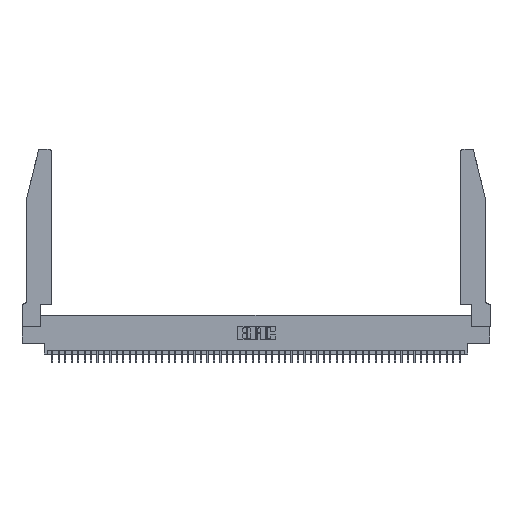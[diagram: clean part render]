
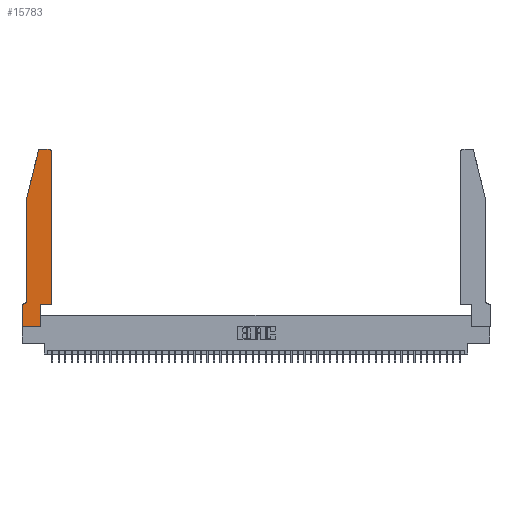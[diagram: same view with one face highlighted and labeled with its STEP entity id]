
A CAD part, top view. The second image highlights one B-rep face of the part: STEP entity #15783.
In plain terms, the highlighted planar face has unit normal (0, 0, 1).
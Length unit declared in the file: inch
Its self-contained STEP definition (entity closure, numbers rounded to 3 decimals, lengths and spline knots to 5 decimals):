
#323 = CARTESIAN_POINT ( 'NONE',  ( 0.284, 2.72, 0.37 ) ) ;
#986 = ORIENTED_EDGE ( 'NONE', *, *, #10492, .T. ) ;
#1044 = EDGE_CURVE ( 'NONE', #39456, #3815, #16891, .T. ) ;
#1156 = VERTEX_POINT ( 'NONE', #30139 ) ;
#1580 = CARTESIAN_POINT ( 'NONE',  ( 0.4505, 2.72, 0.37 ) ) ;
#1683 = CARTESIAN_POINT ( 'NONE',  ( 0.0755, 0.35, 0.37 ) ) ;
#2139 = AXIS2_PLACEMENT_3D ( 'NONE', #43723, #15956, #23377 ) ;
#3011 = PLANE ( 'NONE',  #17793 ) ;
#3158 = VERTEX_POINT ( 'NONE', #9696 ) ;
#3815 = VERTEX_POINT ( 'NONE', #37715 ) ;
#4300 = DIRECTION ( 'NONE',  ( 0., 0., 1. ) ) ;
#5509 = ORIENTED_EDGE ( 'NONE', *, *, #23324, .T. ) ;
#5514 = CIRCLE ( 'NONE', #7210, 0.03 ) ;
#6064 = EDGE_CURVE ( 'NONE', #20552, #37016, #24253, .T. ) ;
#7210 = AXIS2_PLACEMENT_3D ( 'NONE', #323, #4300, #49679 ) ;
#9147 = VERTEX_POINT ( 'NONE', #23112 ) ;
#9696 = CARTESIAN_POINT ( 'NONE',  ( 0.2865, 0.35, 0.37 ) ) ;
#9889 = ORIENTED_EDGE ( 'NONE', *, *, #6064, .T. ) ;
#10321 = VECTOR ( 'NONE', #38450, 39.37008 ) ;
#10492 = EDGE_CURVE ( 'NONE', #1156, #16856, #13989, .T. ) ;
#10498 = CARTESIAN_POINT ( 'NONE',  ( 0.4505, 0.35, 0.37 ) ) ;
#11010 = CARTESIAN_POINT ( 'NONE',  ( 0.2605, 2.75, 0.37 ) ) ;
#11026 = CARTESIAN_POINT ( 'NONE',  ( 0., 0., 0.37 ) ) ;
#11160 = ORIENTED_EDGE ( 'NONE', *, *, #1044, .T. ) ;
#12332 = ORIENTED_EDGE ( 'NONE', *, *, #48215, .T. ) ;
#13614 = VECTOR ( 'NONE', #44052, 39.37008 ) ;
#13898 = LINE ( 'NONE', #26039, #33734 ) ;
#13989 = CIRCLE ( 'NONE', #2139, 0.07 ) ;
#14153 = DIRECTION ( 'NONE',  ( -0.239, -0.971, 0. ) ) ;
#14894 = LINE ( 'NONE', #46168, #40842 ) ;
#15067 = ORIENTED_EDGE ( 'NONE', *, *, #27003, .T. ) ;
#15783 = ADVANCED_FACE ( 'NONE', ( #51404 ), #3011, .T. ) ;
#15956 = DIRECTION ( 'NONE',  ( 0., 0., -1. ) ) ;
#16856 = VERTEX_POINT ( 'NONE', #41423 ) ;
#16891 = CIRCLE ( 'NONE', #51468, 0.03 ) ;
#17680 = CARTESIAN_POINT ( 'NONE',  ( 0.2865, 0., 0.37 ) ) ;
#17793 = AXIS2_PLACEMENT_3D ( 'NONE', #30794, #35275, #31304 ) ;
#20552 = VERTEX_POINT ( 'NONE', #32306 ) ;
#21447 = VECTOR ( 'NONE', #27969, 39.37008 ) ;
#21716 = EDGE_CURVE ( 'NONE', #3158, #40963, #14894, .T. ) ;
#22412 = VERTEX_POINT ( 'NONE', #17680 ) ;
#22620 = VECTOR ( 'NONE', #14153, 39.37008 ) ;
#23112 = CARTESIAN_POINT ( 'NONE',  ( 0.0755, 2., 0.37 ) ) ;
#23324 = EDGE_CURVE ( 'NONE', #40963, #39456, #29226, .T. ) ;
#23377 = DIRECTION ( 'NONE',  ( -1., 0., 0. ) ) ;
#23760 = EDGE_CURVE ( 'NONE', #29981, #45880, #5514, .T. ) ;
#24253 = LINE ( 'NONE', #27253, #45060 ) ;
#24928 = VECTOR ( 'NONE', #45865, 39.37008 ) ;
#26039 = CARTESIAN_POINT ( 'NONE',  ( 0.0755, 2., 0.37 ) ) ;
#26827 = ORIENTED_EDGE ( 'NONE', *, *, #31838, .T. ) ;
#27003 = EDGE_CURVE ( 'NONE', #9147, #1156, #13898, .T. ) ;
#27135 = LINE ( 'NONE', #11010, #13614 ) ;
#27253 = CARTESIAN_POINT ( 'NONE',  ( 0., 0., 0.37 ) ) ;
#27969 = DIRECTION ( 'NONE',  ( 0., 1., 0. ) ) ;
#29226 = LINE ( 'NONE', #41891, #24928 ) ;
#29630 = DIRECTION ( 'NONE',  ( 0., 0., 1. ) ) ;
#29981 = VERTEX_POINT ( 'NONE', #41288 ) ;
#30015 = LINE ( 'NONE', #42165, #22620 ) ;
#30139 = CARTESIAN_POINT ( 'NONE',  ( 0.0755, 0.42, 0.37 ) ) ;
#30794 = CARTESIAN_POINT ( 'NONE',  ( 0., 0.35, 0.37 ) ) ;
#31000 = DIRECTION ( 'NONE',  ( 1., 0., 0. ) ) ;
#31304 = DIRECTION ( 'NONE',  ( 1., 0., 0. ) ) ;
#31838 = EDGE_CURVE ( 'NONE', #22412, #3158, #35647, .T. ) ;
#32297 = ORIENTED_EDGE ( 'NONE', *, *, #38539, .T. ) ;
#32306 = CARTESIAN_POINT ( 'NONE',  ( 0., 0.35, 0.37 ) ) ;
#32815 = ORIENTED_EDGE ( 'NONE', *, *, #46663, .T. ) ;
#33734 = VECTOR ( 'NONE', #38203, 39.37008 ) ;
#33747 = EDGE_CURVE ( 'NONE', #16856, #20552, #38437, .T. ) ;
#34468 = LINE ( 'NONE', #38695, #10321 ) ;
#35275 = DIRECTION ( 'NONE',  ( 0., 0., 1. ) ) ;
#35647 = LINE ( 'NONE', #39588, #21447 ) ;
#37016 = VERTEX_POINT ( 'NONE', #11026 ) ;
#37715 = CARTESIAN_POINT ( 'NONE',  ( 0.4205, 2.75, 0.37 ) ) ;
#38203 = DIRECTION ( 'NONE',  ( 0., -1., 0. ) ) ;
#38437 = LINE ( 'NONE', #1683, #40091 ) ;
#38450 = DIRECTION ( 'NONE',  ( 1., 0., 0. ) ) ;
#38539 = EDGE_CURVE ( 'NONE', #45880, #9147, #30015, .T. ) ;
#38542 = ORIENTED_EDGE ( 'NONE', *, *, #23760, .T. ) ;
#38695 = CARTESIAN_POINT ( 'NONE',  ( 0., 0., 0.37 ) ) ;
#39141 = DIRECTION ( 'NONE',  ( 0., -1., 0. ) ) ;
#39456 = VERTEX_POINT ( 'NONE', #1580 ) ;
#39588 = CARTESIAN_POINT ( 'NONE',  ( 0.2865, 0.35, 0.37 ) ) ;
#40091 = VECTOR ( 'NONE', #41888, 39.37008 ) ;
#40842 = VECTOR ( 'NONE', #31000, 39.37008 ) ;
#40963 = VERTEX_POINT ( 'NONE', #10498 ) ;
#41288 = CARTESIAN_POINT ( 'NONE',  ( 0.284, 2.75, 0.37 ) ) ;
#41423 = CARTESIAN_POINT ( 'NONE',  ( 0.0055, 0.35, 0.37 ) ) ;
#41791 = CARTESIAN_POINT ( 'NONE',  ( 0.4205, 2.72, 0.37 ) ) ;
#41888 = DIRECTION ( 'NONE',  ( -1., 0., 0. ) ) ;
#41891 = CARTESIAN_POINT ( 'NONE',  ( 0.4505, 0.35, 0.37 ) ) ;
#42165 = CARTESIAN_POINT ( 'NONE',  ( 0.0755, 2., 0.37 ) ) ;
#43723 = CARTESIAN_POINT ( 'NONE',  ( 0.0055, 0.42, 0.37 ) ) ;
#44052 = DIRECTION ( 'NONE',  ( -1., 0., 0. ) ) ;
#45060 = VECTOR ( 'NONE', #39141, 39.37008 ) ;
#45241 = ORIENTED_EDGE ( 'NONE', *, *, #21716, .T. ) ;
#45761 = DIRECTION ( 'NONE',  ( 1., 0., 0. ) ) ;
#45865 = DIRECTION ( 'NONE',  ( 0., 1., 0. ) ) ;
#45880 = VERTEX_POINT ( 'NONE', #51584 ) ;
#46168 = CARTESIAN_POINT ( 'NONE',  ( 0.4505, 0.35, 0.37 ) ) ;
#46613 = ORIENTED_EDGE ( 'NONE', *, *, #33747, .T. ) ;
#46663 = EDGE_CURVE ( 'NONE', #3815, #29981, #27135, .T. ) ;
#48215 = EDGE_CURVE ( 'NONE', #37016, #22412, #34468, .T. ) ;
#49679 = DIRECTION ( 'NONE',  ( 1., 0., 0. ) ) ;
#50499 = EDGE_LOOP ( 'NONE', ( #32815, #38542, #32297, #15067, #986, #46613, #9889, #12332, #26827, #45241, #5509, #11160 ) ) ;
#51404 = FACE_OUTER_BOUND ( 'NONE', #50499, .T. ) ;
#51468 = AXIS2_PLACEMENT_3D ( 'NONE', #41791, #29630, #45761 ) ;
#51584 = CARTESIAN_POINT ( 'NONE',  ( 0.25487, 2.72718, 0.37 ) ) ;
